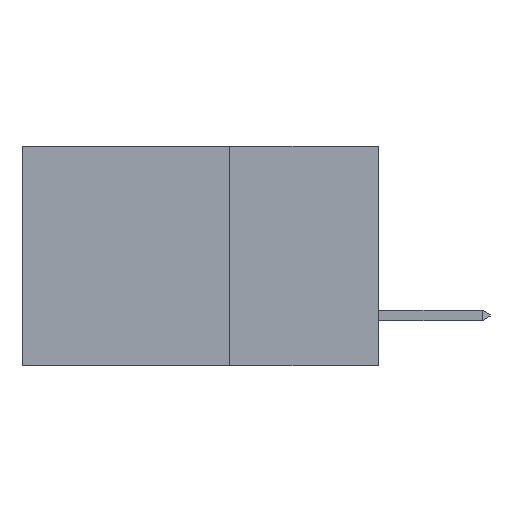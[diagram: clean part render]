
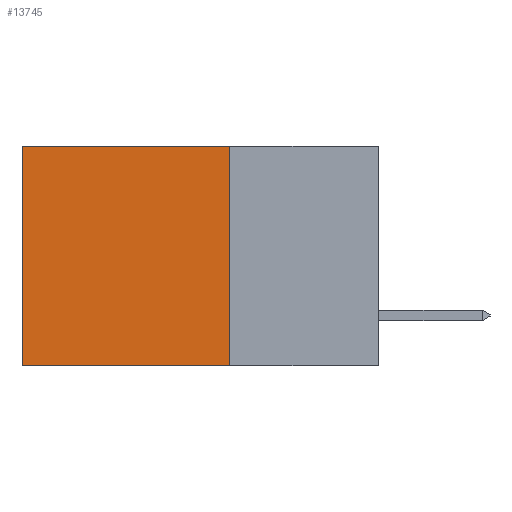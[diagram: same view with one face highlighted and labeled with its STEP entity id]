
A CAD part, left-side view. The second image highlights one B-rep face of the part: STEP entity #13745.
In plain terms, the highlighted planar face has unit normal (-1, 0, 0).
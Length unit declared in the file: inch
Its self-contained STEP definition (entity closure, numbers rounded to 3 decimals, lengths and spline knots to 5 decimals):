
#219 = VERTEX_POINT ( 'NONE', #5098 ) ;
#421 = VERTEX_POINT ( 'NONE', #10933 ) ;
#481 = CARTESIAN_POINT ( 'NONE',  ( 0.2615, 0.25, -0.37 ) ) ;
#1071 = ORIENTED_EDGE ( 'NONE', *, *, #5616, .T. ) ;
#1264 = ORIENTED_EDGE ( 'NONE', *, *, #4239, .T. ) ;
#2230 = VERTEX_POINT ( 'NONE', #4613 ) ;
#2497 = LINE ( 'NONE', #4758, #9064 ) ;
#3035 = FACE_OUTER_BOUND ( 'NONE', #14082, .T. ) ;
#3400 = EDGE_CURVE ( 'NONE', #4729, #421, #12967, .T. ) ;
#3475 = VECTOR ( 'NONE', #15891, 39.37008 ) ;
#4239 = EDGE_CURVE ( 'NONE', #4729, #2230, #7813, .T. ) ;
#4613 = CARTESIAN_POINT ( 'NONE',  ( 0.2615, 0.6, 0. ) ) ;
#4729 = VERTEX_POINT ( 'NONE', #5795 ) ;
#4758 = CARTESIAN_POINT ( 'NONE',  ( 0.2615, 0.25, -0.37 ) ) ;
#4840 = AXIS2_PLACEMENT_3D ( 'NONE', #481, #5884, #14739 ) ;
#5098 = CARTESIAN_POINT ( 'NONE',  ( 0.2615, 0.6, -0.37 ) ) ;
#5616 = EDGE_CURVE ( 'NONE', #2230, #219, #13676, .T. ) ;
#5795 = CARTESIAN_POINT ( 'NONE',  ( 0.2615, 0.25, 0. ) ) ;
#5884 = DIRECTION ( 'NONE',  ( 1., 0., 0. ) ) ;
#6166 = DIRECTION ( 'NONE',  ( 0., 1., 0. ) ) ;
#7813 = LINE ( 'NONE', #16177, #3475 ) ;
#9064 = VECTOR ( 'NONE', #6166, 39.37008 ) ;
#9599 = VECTOR ( 'NONE', #12300, 39.37008 ) ;
#10933 = CARTESIAN_POINT ( 'NONE',  ( 0.2615, 0.25, -0.37 ) ) ;
#11453 = EDGE_CURVE ( 'NONE', #421, #219, #2497, .T. ) ;
#11744 = DIRECTION ( 'NONE',  ( 0., 0., -1. ) ) ;
#11776 = CARTESIAN_POINT ( 'NONE',  ( 0.2615, 0.6, -0.37 ) ) ;
#12300 = DIRECTION ( 'NONE',  ( 0., 0., -1. ) ) ;
#12395 = CARTESIAN_POINT ( 'NONE',  ( 0.2615, 0.25, -0.37 ) ) ;
#12967 = LINE ( 'NONE', #12395, #9599 ) ;
#13287 = VECTOR ( 'NONE', #11744, 39.37008 ) ;
#13484 = PLANE ( 'NONE',  #4840 ) ;
#13676 = LINE ( 'NONE', #11776, #13287 ) ;
#13745 = ADVANCED_FACE ( 'NONE', ( #3035 ), #13484, .F. ) ;
#14082 = EDGE_LOOP ( 'NONE', ( #1071, #16292, #14520, #1264 ) ) ;
#14520 = ORIENTED_EDGE ( 'NONE', *, *, #3400, .F. ) ;
#14739 = DIRECTION ( 'NONE',  ( 0., 0., -1. ) ) ;
#15891 = DIRECTION ( 'NONE',  ( 0., 1., 0. ) ) ;
#16177 = CARTESIAN_POINT ( 'NONE',  ( 0.2615, 0.25, 0. ) ) ;
#16292 = ORIENTED_EDGE ( 'NONE', *, *, #11453, .F. ) ;
